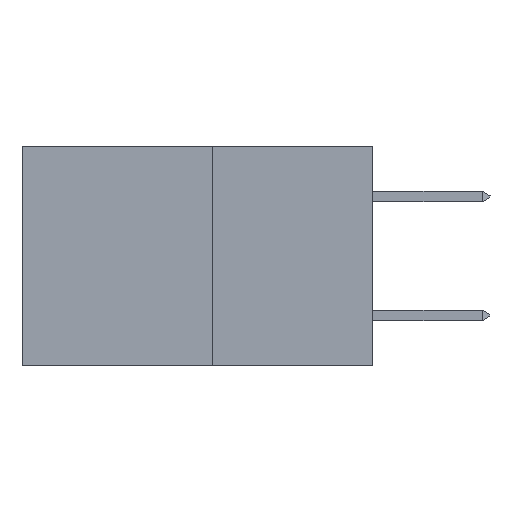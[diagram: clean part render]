
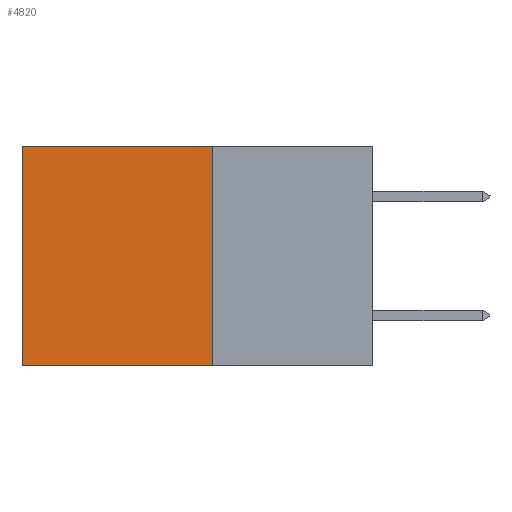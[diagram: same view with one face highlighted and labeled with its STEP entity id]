
A CAD part, left-side view. The second image highlights one B-rep face of the part: STEP entity #4820.
In plain terms, the highlighted planar face has unit normal (-1, 0, 0).
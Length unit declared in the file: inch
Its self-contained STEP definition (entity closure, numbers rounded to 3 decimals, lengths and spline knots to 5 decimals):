
#206 = AXIS2_PLACEMENT_3D ( 'NONE', #3179, #6958, #6852 ) ;
#416 = DIRECTION ( 'NONE',  ( 0., 0., -1. ) ) ;
#1114 = CARTESIAN_POINT ( 'NONE',  ( 0.277, 0.27, 0. ) ) ;
#1589 = CARTESIAN_POINT ( 'NONE',  ( 0.277, 0.27, -0.37 ) ) ;
#1890 = VECTOR ( 'NONE', #416, 39.37008 ) ;
#2050 = DIRECTION ( 'NONE',  ( 0., 1., 0. ) ) ;
#2437 = CARTESIAN_POINT ( 'NONE',  ( 0.277, 0.59, -0.37 ) ) ;
#2555 = DIRECTION ( 'NONE',  ( 0., 1., 0. ) ) ;
#2628 = LINE ( 'NONE', #1589, #17191 ) ;
#2657 = EDGE_CURVE ( 'NONE', #10923, #10122, #12643, .T. ) ;
#2847 = PLANE ( 'NONE',  #206 ) ;
#2989 = EDGE_CURVE ( 'NONE', #5031, #10122, #2628, .T. ) ;
#3140 = EDGE_LOOP ( 'NONE', ( #9691, #6056, #10847, #11358 ) ) ;
#3179 = CARTESIAN_POINT ( 'NONE',  ( 0.277, 0.27, -0.37 ) ) ;
#4625 = CARTESIAN_POINT ( 'NONE',  ( 0.277, 0.27, -0.37 ) ) ;
#4756 = CARTESIAN_POINT ( 'NONE',  ( 0.277, 0.27, -0.37 ) ) ;
#4820 = ADVANCED_FACE ( 'NONE', ( #6389 ), #2847, .F. ) ;
#5031 = VERTEX_POINT ( 'NONE', #4625 ) ;
#5251 = CARTESIAN_POINT ( 'NONE',  ( 0.277, 0.59, -0.37 ) ) ;
#6056 = ORIENTED_EDGE ( 'NONE', *, *, #2989, .F. ) ;
#6389 = FACE_OUTER_BOUND ( 'NONE', #3140, .T. ) ;
#6852 = DIRECTION ( 'NONE',  ( 0., 0., -1. ) ) ;
#6958 = DIRECTION ( 'NONE',  ( 1., 0., 0. ) ) ;
#7311 = LINE ( 'NONE', #1114, #14357 ) ;
#8484 = VECTOR ( 'NONE', #18026, 39.37008 ) ;
#9103 = CARTESIAN_POINT ( 'NONE',  ( 0.277, 0.27, 0. ) ) ;
#9691 = ORIENTED_EDGE ( 'NONE', *, *, #2657, .T. ) ;
#10122 = VERTEX_POINT ( 'NONE', #5251 ) ;
#10633 = VERTEX_POINT ( 'NONE', #9103 ) ;
#10847 = ORIENTED_EDGE ( 'NONE', *, *, #14293, .F. ) ;
#10923 = VERTEX_POINT ( 'NONE', #11144 ) ;
#11144 = CARTESIAN_POINT ( 'NONE',  ( 0.277, 0.59, 0. ) ) ;
#11358 = ORIENTED_EDGE ( 'NONE', *, *, #12105, .T. ) ;
#12105 = EDGE_CURVE ( 'NONE', #10633, #10923, #7311, .T. ) ;
#12643 = LINE ( 'NONE', #2437, #8484 ) ;
#14293 = EDGE_CURVE ( 'NONE', #10633, #5031, #16497, .T. ) ;
#14357 = VECTOR ( 'NONE', #2555, 39.37008 ) ;
#16497 = LINE ( 'NONE', #4756, #1890 ) ;
#17191 = VECTOR ( 'NONE', #2050, 39.37008 ) ;
#18026 = DIRECTION ( 'NONE',  ( 0., 0., -1. ) ) ;
